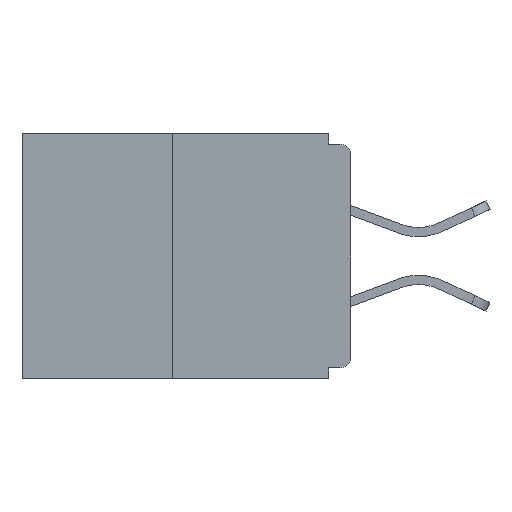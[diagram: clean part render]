
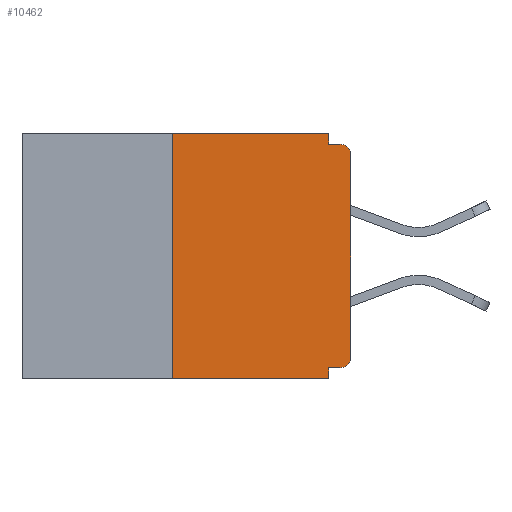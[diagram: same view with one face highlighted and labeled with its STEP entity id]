
A CAD part, left-side view. The second image highlights one B-rep face of the part: STEP entity #10462.
In plain terms, the highlighted planar face has unit normal (-1, 0, 0).
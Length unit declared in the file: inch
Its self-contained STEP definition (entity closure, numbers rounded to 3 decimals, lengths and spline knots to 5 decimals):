
#59 = CARTESIAN_POINT ( 'NONE',  ( 0., 0.031, -0.328 ) ) ;
#88 = DIRECTION ( 'NONE',  ( 0., 1., 0. ) ) ;
#112 = VECTOR ( 'NONE', #17438, 39.37008 ) ;
#673 = LINE ( 'NONE', #10920, #9469 ) ;
#831 = CARTESIAN_POINT ( 'NONE',  ( 0., 0.46, 0. ) ) ;
#1074 = ORIENTED_EDGE ( 'NONE', *, *, #14580, .F. ) ;
#1089 = CARTESIAN_POINT ( 'NONE',  ( 0., 0.015, -0.313 ) ) ;
#1517 = ORIENTED_EDGE ( 'NONE', *, *, #10909, .T. ) ;
#1646 = VERTEX_POINT ( 'NONE', #16431 ) ;
#1710 = CARTESIAN_POINT ( 'NONE',  ( 0., 0.015, -0.328 ) ) ;
#3413 = DIRECTION ( 'NONE',  ( 0., 0., -1. ) ) ;
#3437 = EDGE_CURVE ( 'NONE', #3715, #16677, #14314, .T. ) ;
#3715 = VERTEX_POINT ( 'NONE', #10993 ) ;
#3735 = DIRECTION ( 'NONE',  ( 0., 0., -1. ) ) ;
#3855 = ORIENTED_EDGE ( 'NONE', *, *, #9117, .F. ) ;
#3952 = DIRECTION ( 'NONE',  ( 0., -1., 0. ) ) ;
#4402 = CARTESIAN_POINT ( 'NONE',  ( 0., 0., -0.328 ) ) ;
#4513 = DIRECTION ( 'NONE',  ( 0., -1., 0. ) ) ;
#4650 = DIRECTION ( 'NONE',  ( -1., 0., 0. ) ) ;
#5052 = ORIENTED_EDGE ( 'NONE', *, *, #3437, .F. ) ;
#5345 = LINE ( 'NONE', #7267, #11824 ) ;
#5812 = CIRCLE ( 'NONE', #9684, 0.015 ) ;
#6756 = VERTEX_POINT ( 'NONE', #59 ) ;
#7188 = VERTEX_POINT ( 'NONE', #1710 ) ;
#7223 = DIRECTION ( 'NONE',  ( 0., -1., 0. ) ) ;
#7242 = ORIENTED_EDGE ( 'NONE', *, *, #12900, .F. ) ;
#7267 = CARTESIAN_POINT ( 'NONE',  ( 0., 0., 0. ) ) ;
#7548 = LINE ( 'NONE', #12015, #8627 ) ;
#7563 = ORIENTED_EDGE ( 'NONE', *, *, #12128, .F. ) ;
#7594 = CARTESIAN_POINT ( 'NONE',  ( 0., 0.015, -0.03 ) ) ;
#7689 = ORIENTED_EDGE ( 'NONE', *, *, #14406, .T. ) ;
#7799 = PLANE ( 'NONE',  #11016 ) ;
#8315 = EDGE_CURVE ( 'NONE', #17437, #14229, #5345, .T. ) ;
#8433 = VECTOR ( 'NONE', #7223, 39.37008 ) ;
#8533 = LINE ( 'NONE', #14662, #8760 ) ;
#8594 = CARTESIAN_POINT ( 'NONE',  ( 0., 0.031, -0.015 ) ) ;
#8627 = VECTOR ( 'NONE', #3952, 39.37008 ) ;
#8760 = VECTOR ( 'NONE', #14501, 39.37008 ) ;
#9117 = EDGE_CURVE ( 'NONE', #6756, #9168, #8533, .T. ) ;
#9165 = AXIS2_PLACEMENT_3D ( 'NONE', #7594, #4650, #3413 ) ;
#9168 = VERTEX_POINT ( 'NONE', #13418 ) ;
#9272 = CARTESIAN_POINT ( 'NONE',  ( 0., 0., -0.313 ) ) ;
#9469 = VECTOR ( 'NONE', #9675, 39.37008 ) ;
#9568 = ORIENTED_EDGE ( 'NONE', *, *, #8315, .T. ) ;
#9675 = DIRECTION ( 'NONE',  ( 0., 0., -1. ) ) ;
#9684 = AXIS2_PLACEMENT_3D ( 'NONE', #1089, #10702, #3735 ) ;
#9773 = VECTOR ( 'NONE', #4513, 39.37008 ) ;
#10462 = ADVANCED_FACE ( 'NONE', ( #11136 ), #7799, .F. ) ;
#10517 = DIRECTION ( 'NONE',  ( 0., 0., -1. ) ) ;
#10702 = DIRECTION ( 'NONE',  ( -1., 0., 0. ) ) ;
#10909 = EDGE_CURVE ( 'NONE', #14229, #13568, #14985, .T. ) ;
#10920 = CARTESIAN_POINT ( 'NONE',  ( 0., 0.031, 0. ) ) ;
#10993 = CARTESIAN_POINT ( 'NONE',  ( 0., 0.25, -0.343 ) ) ;
#11016 = AXIS2_PLACEMENT_3D ( 'NONE', #831, #13127, #10517 ) ;
#11136 = FACE_OUTER_BOUND ( 'NONE', #11514, .T. ) ;
#11514 = EDGE_LOOP ( 'NONE', ( #15930, #5052, #7689, #3855, #7242, #15799, #9568, #1517, #7563, #1074 ) ) ;
#11541 = CARTESIAN_POINT ( 'NONE',  ( 0., 0.25, 0. ) ) ;
#11824 = VECTOR ( 'NONE', #17277, 39.37008 ) ;
#11910 = VECTOR ( 'NONE', #88, 39.37008 ) ;
#12015 = CARTESIAN_POINT ( 'NONE',  ( 0., 0.46, -0.343 ) ) ;
#12128 = EDGE_CURVE ( 'NONE', #16439, #13568, #17532, .T. ) ;
#12724 = CARTESIAN_POINT ( 'NONE',  ( 0., 0.46, 0. ) ) ;
#12900 = EDGE_CURVE ( 'NONE', #7188, #6756, #13837, .T. ) ;
#12992 = LINE ( 'NONE', #12724, #8433 ) ;
#13040 = EDGE_CURVE ( 'NONE', #16677, #1646, #12992, .T. ) ;
#13127 = DIRECTION ( 'NONE',  ( 1., 0., 0. ) ) ;
#13310 = CARTESIAN_POINT ( 'NONE',  ( 0., 0., -0.03 ) ) ;
#13418 = CARTESIAN_POINT ( 'NONE',  ( 0., 0.031, -0.343 ) ) ;
#13568 = VERTEX_POINT ( 'NONE', #14851 ) ;
#13837 = LINE ( 'NONE', #4402, #11910 ) ;
#14229 = VERTEX_POINT ( 'NONE', #13310 ) ;
#14236 = EDGE_CURVE ( 'NONE', #7188, #17437, #5812, .T. ) ;
#14314 = LINE ( 'NONE', #17389, #112 ) ;
#14406 = EDGE_CURVE ( 'NONE', #3715, #9168, #7548, .T. ) ;
#14501 = DIRECTION ( 'NONE',  ( 0., 0., -1. ) ) ;
#14580 = EDGE_CURVE ( 'NONE', #1646, #16439, #673, .T. ) ;
#14662 = CARTESIAN_POINT ( 'NONE',  ( 0., 0.031, -0.343 ) ) ;
#14851 = CARTESIAN_POINT ( 'NONE',  ( 0., 0.015, -0.015 ) ) ;
#14985 = CIRCLE ( 'NONE', #9165, 0.015 ) ;
#15799 = ORIENTED_EDGE ( 'NONE', *, *, #14236, .T. ) ;
#15930 = ORIENTED_EDGE ( 'NONE', *, *, #13040, .F. ) ;
#16431 = CARTESIAN_POINT ( 'NONE',  ( 0., 0.031, 0. ) ) ;
#16439 = VERTEX_POINT ( 'NONE', #8594 ) ;
#16677 = VERTEX_POINT ( 'NONE', #11541 ) ;
#17185 = CARTESIAN_POINT ( 'NONE',  ( 0., 0., -0.015 ) ) ;
#17277 = DIRECTION ( 'NONE',  ( 0., 0., 1. ) ) ;
#17389 = CARTESIAN_POINT ( 'NONE',  ( 0., 0.25, 0. ) ) ;
#17437 = VERTEX_POINT ( 'NONE', #9272 ) ;
#17438 = DIRECTION ( 'NONE',  ( 0., 0., 1. ) ) ;
#17532 = LINE ( 'NONE', #17185, #9773 ) ;
